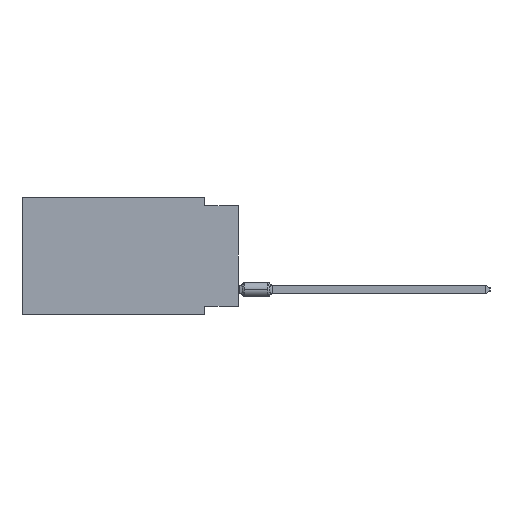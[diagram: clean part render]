
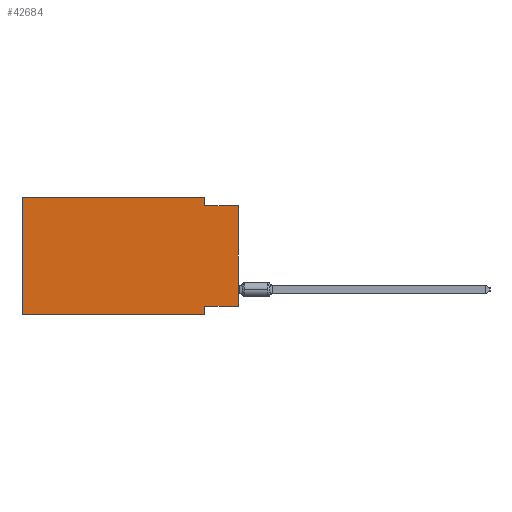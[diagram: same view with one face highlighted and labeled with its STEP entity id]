
A CAD part, left-side view. The second image highlights one B-rep face of the part: STEP entity #42684.
In plain terms, the highlighted planar face has unit normal (-1, 0, 0).
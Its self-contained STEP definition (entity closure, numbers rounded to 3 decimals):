
#201 = ORIENTED_EDGE ( 'NONE', *, *, #6411, .F. ) ;
#226 = VERTEX_POINT ( 'NONE', #50737 ) ;
#1313 = DIRECTION ( 'NONE',  ( 0., 0., 1. ) ) ;
#2484 = DIRECTION ( 'NONE',  ( 0., 0., -1. ) ) ;
#4658 = CARTESIAN_POINT ( 'NONE',  ( 0., 2.54, -0.635 ) ) ;
#6071 = VECTOR ( 'NONE', #69538, 1000. ) ;
#6411 = EDGE_CURVE ( 'NONE', #63208, #46600, #17120, .T. ) ;
#6961 = LINE ( 'NONE', #35108, #42658 ) ;
#9349 = CARTESIAN_POINT ( 'NONE',  ( 0., 16.383, 0. ) ) ;
#9848 = CARTESIAN_POINT ( 'NONE',  ( 0., 16.383, 0. ) ) ;
#12295 = CARTESIAN_POINT ( 'NONE',  ( 0., 0., 0. ) ) ;
#13280 = LINE ( 'NONE', #35579, #6071 ) ;
#13289 = EDGE_LOOP ( 'NONE', ( #55913, #33144, #29013, #16812, #51750, #20536, #22410, #201 ) ) ;
#14795 = VERTEX_POINT ( 'NONE', #4658 ) ;
#15045 = EDGE_CURVE ( 'NONE', #35157, #43183, #19956, .T. ) ;
#15204 = EDGE_CURVE ( 'NONE', #29030, #57209, #49886, .T. ) ;
#15554 = DIRECTION ( 'NONE',  ( 0., -1., 0. ) ) ;
#16033 = CARTESIAN_POINT ( 'NONE',  ( 0., 0., -8.255 ) ) ;
#16812 = ORIENTED_EDGE ( 'NONE', *, *, #15045, .F. ) ;
#17044 = DIRECTION ( 'NONE',  ( 0., 0., -1. ) ) ;
#17120 = LINE ( 'NONE', #16033, #48851 ) ;
#18761 = EDGE_CURVE ( 'NONE', #14795, #226, #6961, .T. ) ;
#18776 = VECTOR ( 'NONE', #58309, 1000. ) ;
#19956 = LINE ( 'NONE', #9349, #66848 ) ;
#20470 = EDGE_CURVE ( 'NONE', #46600, #57209, #29942, .T. ) ;
#20536 = ORIENTED_EDGE ( 'NONE', *, *, #15204, .T. ) ;
#22410 = ORIENTED_EDGE ( 'NONE', *, *, #20470, .F. ) ;
#24011 = LINE ( 'NONE', #12295, #36163 ) ;
#24413 = EDGE_CURVE ( 'NONE', #63208, #226, #24011, .T. ) ;
#24905 = VECTOR ( 'NONE', #15554, 1000. ) ;
#25166 = CARTESIAN_POINT ( 'NONE',  ( 0., 2.54, -8.89 ) ) ;
#27752 = CARTESIAN_POINT ( 'NONE',  ( 0., 2.54, -8.255 ) ) ;
#29013 = ORIENTED_EDGE ( 'NONE', *, *, #36087, .F. ) ;
#29030 = VERTEX_POINT ( 'NONE', #55985 ) ;
#29648 = DIRECTION ( 'NONE',  ( 0., -1., 0. ) ) ;
#29942 = LINE ( 'NONE', #25166, #40600 ) ;
#33144 = ORIENTED_EDGE ( 'NONE', *, *, #18761, .F. ) ;
#33496 = PLANE ( 'NONE',  #54425 ) ;
#34920 = CARTESIAN_POINT ( 'NONE',  ( 0., 16.383, 0. ) ) ;
#35108 = CARTESIAN_POINT ( 'NONE',  ( 0., 0., -0.635 ) ) ;
#35157 = VERTEX_POINT ( 'NONE', #9848 ) ;
#35579 = CARTESIAN_POINT ( 'NONE',  ( 0., 16.383, 0. ) ) ;
#36087 = EDGE_CURVE ( 'NONE', #43183, #14795, #68162, .T. ) ;
#36163 = VECTOR ( 'NONE', #1313, 1000. ) ;
#38832 = EDGE_CURVE ( 'NONE', #29030, #35157, #13280, .T. ) ;
#40600 = VECTOR ( 'NONE', #2484, 1000. ) ;
#42658 = VECTOR ( 'NONE', #29648, 1000. ) ;
#42684 = ADVANCED_FACE ( 'NONE', ( #49914 ), #33496, .F. ) ;
#43183 = VERTEX_POINT ( 'NONE', #67978 ) ;
#45157 = DIRECTION ( 'NONE',  ( 1., 0., 0. ) ) ;
#46600 = VERTEX_POINT ( 'NONE', #27752 ) ;
#48851 = VECTOR ( 'NONE', #66440, 1000. ) ;
#49886 = LINE ( 'NONE', #60120, #24905 ) ;
#49914 = FACE_OUTER_BOUND ( 'NONE', #13289, .T. ) ;
#50737 = CARTESIAN_POINT ( 'NONE',  ( 0., 0., -0.635 ) ) ;
#51408 = CARTESIAN_POINT ( 'NONE',  ( 0., 0., -8.255 ) ) ;
#51750 = ORIENTED_EDGE ( 'NONE', *, *, #38832, .F. ) ;
#54425 = AXIS2_PLACEMENT_3D ( 'NONE', #34920, #45157, #17044 ) ;
#55913 = ORIENTED_EDGE ( 'NONE', *, *, #24413, .T. ) ;
#55985 = CARTESIAN_POINT ( 'NONE',  ( 0., 16.383, -8.89 ) ) ;
#57209 = VERTEX_POINT ( 'NONE', #70390 ) ;
#57957 = CARTESIAN_POINT ( 'NONE',  ( 0., 2.54, 0. ) ) ;
#58309 = DIRECTION ( 'NONE',  ( 0., 0., -1. ) ) ;
#60120 = CARTESIAN_POINT ( 'NONE',  ( 0., 16.383, -8.89 ) ) ;
#63208 = VERTEX_POINT ( 'NONE', #51408 ) ;
#66440 = DIRECTION ( 'NONE',  ( 0., 1., 0. ) ) ;
#66848 = VECTOR ( 'NONE', #70006, 1000. ) ;
#67978 = CARTESIAN_POINT ( 'NONE',  ( 0., 2.54, 0. ) ) ;
#68162 = LINE ( 'NONE', #57957, #18776 ) ;
#69538 = DIRECTION ( 'NONE',  ( 0., 0., 1. ) ) ;
#70006 = DIRECTION ( 'NONE',  ( 0., -1., 0. ) ) ;
#70390 = CARTESIAN_POINT ( 'NONE',  ( 0., 2.54, -8.89 ) ) ;
